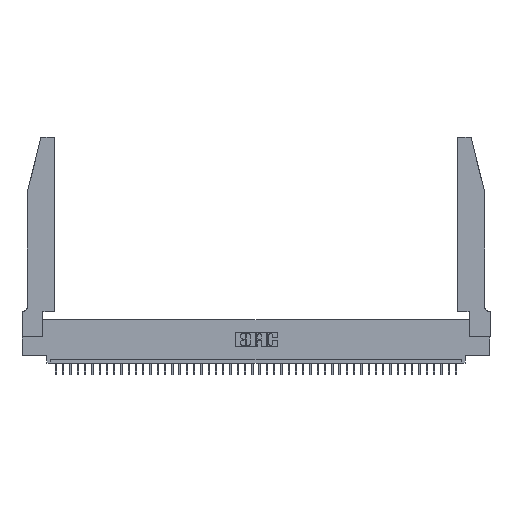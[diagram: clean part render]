
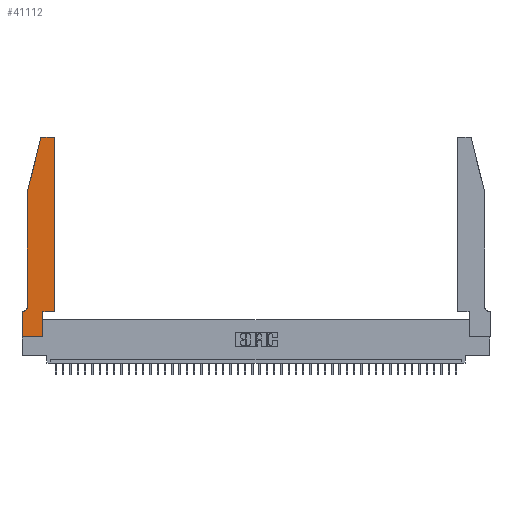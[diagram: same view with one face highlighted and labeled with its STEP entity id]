
A CAD part, top view. The second image highlights one B-rep face of the part: STEP entity #41112.
In plain terms, the highlighted planar face has unit normal (0, 0, 1).
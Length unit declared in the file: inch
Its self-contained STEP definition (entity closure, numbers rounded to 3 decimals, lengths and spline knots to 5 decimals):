
#143 = VERTEX_POINT ( 'NONE', #19541 ) ;
#1109 = AXIS2_PLACEMENT_3D ( 'NONE', #14229, #17727, #10408 ) ;
#1796 = ORIENTED_EDGE ( 'NONE', *, *, #12686, .T. ) ;
#1895 = VERTEX_POINT ( 'NONE', #22024 ) ;
#2166 = VECTOR ( 'NONE', #28571, 39.37008 ) ;
#2323 = CARTESIAN_POINT ( 'NONE',  ( 0., 0., 0.37 ) ) ;
#2516 = LINE ( 'NONE', #33972, #38517 ) ;
#2550 = CARTESIAN_POINT ( 'NONE',  ( 0.0755, 2., 0.37 ) ) ;
#2597 = DIRECTION ( 'NONE',  ( 1., 0., 0. ) ) ;
#3329 = PLANE ( 'NONE',  #1109 ) ;
#6691 = DIRECTION ( 'NONE',  ( 0., 0., 1. ) ) ;
#7042 = EDGE_CURVE ( 'NONE', #10030, #10248, #19528, .T. ) ;
#7094 = AXIS2_PLACEMENT_3D ( 'NONE', #9992, #17031, #23874 ) ;
#7637 = LINE ( 'NONE', #10765, #2166 ) ;
#7688 = EDGE_CURVE ( 'NONE', #40083, #19328, #18351, .T. ) ;
#8782 = VECTOR ( 'NONE', #24478, 39.37008 ) ;
#9147 = VERTEX_POINT ( 'NONE', #32725 ) ;
#9392 = VERTEX_POINT ( 'NONE', #40811 ) ;
#9992 = CARTESIAN_POINT ( 'NONE',  ( 0.0055, 0.42, 0.37 ) ) ;
#10030 = VERTEX_POINT ( 'NONE', #20169 ) ;
#10248 = VERTEX_POINT ( 'NONE', #20883 ) ;
#10408 = DIRECTION ( 'NONE',  ( 1., 0., 0. ) ) ;
#10765 = CARTESIAN_POINT ( 'NONE',  ( 0., 0., 0.37 ) ) ;
#10864 = EDGE_LOOP ( 'NONE', ( #1796, #42692, #13983, #28586, #14990, #34557, #24993, #42675, #35325, #22037, #21359, #24516 ) ) ;
#11516 = DIRECTION ( 'NONE',  ( -1., 0., 0. ) ) ;
#12686 = EDGE_CURVE ( 'NONE', #19328, #20302, #2516, .T. ) ;
#12767 = DIRECTION ( 'NONE',  ( 0., -1., 0. ) ) ;
#13983 = ORIENTED_EDGE ( 'NONE', *, *, #7042, .T. ) ;
#14229 = CARTESIAN_POINT ( 'NONE',  ( 0., 0.35, 0.37 ) ) ;
#14476 = CIRCLE ( 'NONE', #7094, 0.07 ) ;
#14661 = AXIS2_PLACEMENT_3D ( 'NONE', #27606, #6691, #27338 ) ;
#14990 = ORIENTED_EDGE ( 'NONE', *, *, #21992, .T. ) ;
#15449 = FACE_OUTER_BOUND ( 'NONE', #10864, .T. ) ;
#15538 = CARTESIAN_POINT ( 'NONE',  ( 0.284, 2.75, 0.37 ) ) ;
#15707 = DIRECTION ( 'NONE',  ( 0., 0., 1. ) ) ;
#16818 = VERTEX_POINT ( 'NONE', #41411 ) ;
#17031 = DIRECTION ( 'NONE',  ( 0., 0., -1. ) ) ;
#17643 = EDGE_CURVE ( 'NONE', #9392, #1895, #25584, .T. ) ;
#17727 = DIRECTION ( 'NONE',  ( 0., 0., 1. ) ) ;
#18129 = VERTEX_POINT ( 'NONE', #24982 ) ;
#18351 = CIRCLE ( 'NONE', #33491, 0.03 ) ;
#18427 = VECTOR ( 'NONE', #11516, 39.37008 ) ;
#18517 = VECTOR ( 'NONE', #27286, 39.37008 ) ;
#19143 = VECTOR ( 'NONE', #2597, 39.37008 ) ;
#19328 = VERTEX_POINT ( 'NONE', #25187 ) ;
#19482 = EDGE_CURVE ( 'NONE', #1895, #16818, #7637, .T. ) ;
#19528 = LINE ( 'NONE', #2550, #24957 ) ;
#19541 = CARTESIAN_POINT ( 'NONE',  ( 0.4505, 0.35, 0.37 ) ) ;
#19932 = EDGE_CURVE ( 'NONE', #143, #40083, #26748, .T. ) ;
#20169 = CARTESIAN_POINT ( 'NONE',  ( 0.25487, 2.72718, 0.37 ) ) ;
#20302 = VERTEX_POINT ( 'NONE', #15538 ) ;
#20305 = CARTESIAN_POINT ( 'NONE',  ( 0.4205, 2.72, 0.37 ) ) ;
#20883 = CARTESIAN_POINT ( 'NONE',  ( 0.0755, 2., 0.37 ) ) ;
#21359 = ORIENTED_EDGE ( 'NONE', *, *, #19932, .T. ) ;
#21938 = DIRECTION ( 'NONE',  ( 0., -1., 0. ) ) ;
#21992 = EDGE_CURVE ( 'NONE', #18129, #38800, #14476, .T. ) ;
#22024 = CARTESIAN_POINT ( 'NONE',  ( 0., 0., 0.37 ) ) ;
#22037 = ORIENTED_EDGE ( 'NONE', *, *, #24668, .T. ) ;
#23874 = DIRECTION ( 'NONE',  ( -1., 0., 0. ) ) ;
#24181 = CARTESIAN_POINT ( 'NONE',  ( 0.2865, 0.35, 0.37 ) ) ;
#24478 = DIRECTION ( 'NONE',  ( 0., 1., 0. ) ) ;
#24516 = ORIENTED_EDGE ( 'NONE', *, *, #7688, .T. ) ;
#24668 = EDGE_CURVE ( 'NONE', #9147, #143, #43100, .T. ) ;
#24957 = VECTOR ( 'NONE', #30057, 39.37008 ) ;
#24982 = CARTESIAN_POINT ( 'NONE',  ( 0.0755, 0.42, 0.37 ) ) ;
#24993 = ORIENTED_EDGE ( 'NONE', *, *, #17643, .T. ) ;
#25187 = CARTESIAN_POINT ( 'NONE',  ( 0.4205, 2.75, 0.37 ) ) ;
#25224 = CARTESIAN_POINT ( 'NONE',  ( 0.0755, 0.35, 0.37 ) ) ;
#25584 = LINE ( 'NONE', #2323, #29336 ) ;
#26748 = LINE ( 'NONE', #41405, #18517 ) ;
#26998 = DIRECTION ( 'NONE',  ( 1., 0., 0. ) ) ;
#27157 = VECTOR ( 'NONE', #21938, 39.37008 ) ;
#27286 = DIRECTION ( 'NONE',  ( 0., 1., 0. ) ) ;
#27338 = DIRECTION ( 'NONE',  ( 1., 0., 0. ) ) ;
#27606 = CARTESIAN_POINT ( 'NONE',  ( 0.284, 2.72, 0.37 ) ) ;
#28571 = DIRECTION ( 'NONE',  ( 1., 0., 0. ) ) ;
#28586 = ORIENTED_EDGE ( 'NONE', *, *, #44714, .T. ) ;
#28778 = CARTESIAN_POINT ( 'NONE',  ( 0.0755, 2., 0.37 ) ) ;
#29336 = VECTOR ( 'NONE', #12767, 39.37008 ) ;
#30020 = LINE ( 'NONE', #24181, #8782 ) ;
#30057 = DIRECTION ( 'NONE',  ( -0.239, -0.971, 0. ) ) ;
#31683 = EDGE_CURVE ( 'NONE', #20302, #10030, #36496, .T. ) ;
#32725 = CARTESIAN_POINT ( 'NONE',  ( 0.2865, 0.35, 0.37 ) ) ;
#33491 = AXIS2_PLACEMENT_3D ( 'NONE', #20305, #15707, #26998 ) ;
#33972 = CARTESIAN_POINT ( 'NONE',  ( 0.2605, 2.75, 0.37 ) ) ;
#34114 = DIRECTION ( 'NONE',  ( -1., 0., 0. ) ) ;
#34294 = EDGE_CURVE ( 'NONE', #38800, #9392, #36983, .T. ) ;
#34557 = ORIENTED_EDGE ( 'NONE', *, *, #34294, .T. ) ;
#35325 = ORIENTED_EDGE ( 'NONE', *, *, #42250, .T. ) ;
#35804 = LINE ( 'NONE', #28778, #27157 ) ;
#36496 = CIRCLE ( 'NONE', #14661, 0.03 ) ;
#36983 = LINE ( 'NONE', #25224, #18427 ) ;
#38517 = VECTOR ( 'NONE', #34114, 39.37008 ) ;
#38800 = VERTEX_POINT ( 'NONE', #40979 ) ;
#40083 = VERTEX_POINT ( 'NONE', #42462 ) ;
#40582 = CARTESIAN_POINT ( 'NONE',  ( 0.4505, 0.35, 0.37 ) ) ;
#40811 = CARTESIAN_POINT ( 'NONE',  ( 0., 0.35, 0.37 ) ) ;
#40979 = CARTESIAN_POINT ( 'NONE',  ( 0.0055, 0.35, 0.37 ) ) ;
#41112 = ADVANCED_FACE ( 'NONE', ( #15449 ), #3329, .T. ) ;
#41405 = CARTESIAN_POINT ( 'NONE',  ( 0.4505, 0.35, 0.37 ) ) ;
#41411 = CARTESIAN_POINT ( 'NONE',  ( 0.2865, 0., 0.37 ) ) ;
#42250 = EDGE_CURVE ( 'NONE', #16818, #9147, #30020, .T. ) ;
#42462 = CARTESIAN_POINT ( 'NONE',  ( 0.4505, 2.72, 0.37 ) ) ;
#42675 = ORIENTED_EDGE ( 'NONE', *, *, #19482, .T. ) ;
#42692 = ORIENTED_EDGE ( 'NONE', *, *, #31683, .T. ) ;
#43100 = LINE ( 'NONE', #40582, #19143 ) ;
#44714 = EDGE_CURVE ( 'NONE', #10248, #18129, #35804, .T. ) ;
